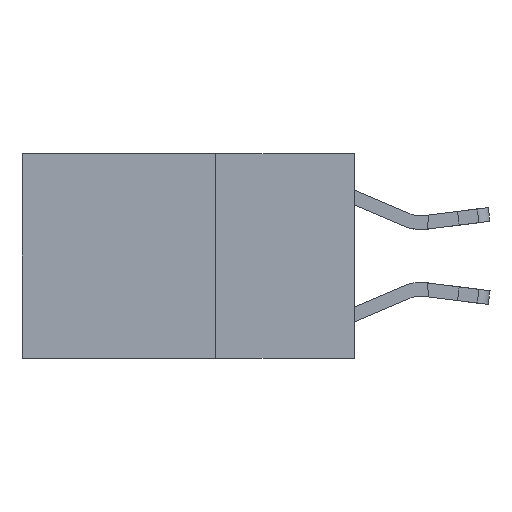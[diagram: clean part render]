
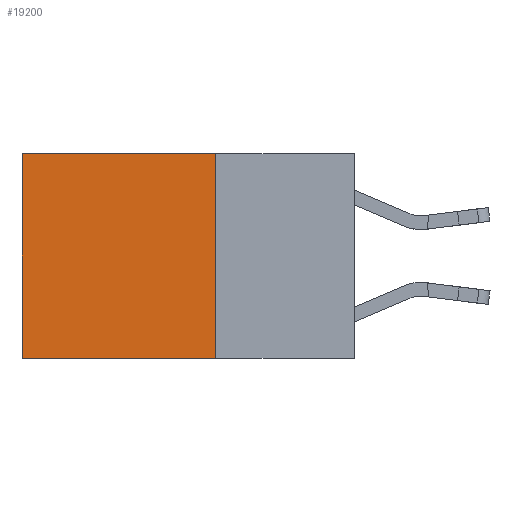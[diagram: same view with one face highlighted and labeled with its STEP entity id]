
A CAD part, left-side view. The second image highlights one B-rep face of the part: STEP entity #19200.
In plain terms, the highlighted planar face has unit normal (-1, 0, 0).
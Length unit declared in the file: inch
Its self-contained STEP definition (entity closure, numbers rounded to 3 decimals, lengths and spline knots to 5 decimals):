
#217 = CARTESIAN_POINT ( 'NONE',  ( 0.2625, 0.6, 0. ) ) ;
#362 = VERTEX_POINT ( 'NONE', #217 ) ;
#408 = VERTEX_POINT ( 'NONE', #25054 ) ;
#1360 = VERTEX_POINT ( 'NONE', #9337 ) ;
#1453 = ORIENTED_EDGE ( 'NONE', *, *, #7594, .F. ) ;
#2041 = CARTESIAN_POINT ( 'NONE',  ( 0.2625, 0.6, 0. ) ) ;
#2956 = DIRECTION ( 'NONE',  ( 0., 1., 0. ) ) ;
#3911 = CARTESIAN_POINT ( 'NONE',  ( 0.2625, 0.25, -0.37 ) ) ;
#4920 = PLANE ( 'NONE',  #14496 ) ;
#5156 = EDGE_CURVE ( 'NONE', #1360, #13276, #16304, .T. ) ;
#5285 = VECTOR ( 'NONE', #17601, 39.37008 ) ;
#6774 = CARTESIAN_POINT ( 'NONE',  ( 0.2625, 0.25, 0. ) ) ;
#6838 = LINE ( 'NONE', #7278, #8966 ) ;
#7278 = CARTESIAN_POINT ( 'NONE',  ( 0.2625, 0.25, 0. ) ) ;
#7594 = EDGE_CURVE ( 'NONE', #408, #1360, #13729, .T. ) ;
#8145 = EDGE_CURVE ( 'NONE', #408, #362, #6838, .T. ) ;
#8325 = ORIENTED_EDGE ( 'NONE', *, *, #8145, .T. ) ;
#8966 = VECTOR ( 'NONE', #2956, 39.37008 ) ;
#8975 = FACE_OUTER_BOUND ( 'NONE', #25027, .T. ) ;
#9202 = DIRECTION ( 'NONE',  ( 0., 1., 0. ) ) ;
#9337 = CARTESIAN_POINT ( 'NONE',  ( 0.2625, 0.25, -0.37 ) ) ;
#11284 = LINE ( 'NONE', #2041, #5285 ) ;
#13276 = VERTEX_POINT ( 'NONE', #14331 ) ;
#13729 = LINE ( 'NONE', #23953, #22444 ) ;
#13831 = DIRECTION ( 'NONE',  ( 0., 0., -1. ) ) ;
#14331 = CARTESIAN_POINT ( 'NONE',  ( 0.2625, 0.6, -0.37 ) ) ;
#14496 = AXIS2_PLACEMENT_3D ( 'NONE', #6774, #27207, #13831 ) ;
#16304 = LINE ( 'NONE', #3911, #20131 ) ;
#17024 = ORIENTED_EDGE ( 'NONE', *, *, #24346, .T. ) ;
#17601 = DIRECTION ( 'NONE',  ( 0., 0., -1. ) ) ;
#19200 = ADVANCED_FACE ( 'NONE', ( #8975 ), #4920, .F. ) ;
#20131 = VECTOR ( 'NONE', #9202, 39.37008 ) ;
#21821 = DIRECTION ( 'NONE',  ( 0., 0., -1. ) ) ;
#22444 = VECTOR ( 'NONE', #21821, 39.37008 ) ;
#23953 = CARTESIAN_POINT ( 'NONE',  ( 0.2625, 0.25, 0. ) ) ;
#24346 = EDGE_CURVE ( 'NONE', #362, #13276, #11284, .T. ) ;
#25027 = EDGE_LOOP ( 'NONE', ( #17024, #27719, #1453, #8325 ) ) ;
#25054 = CARTESIAN_POINT ( 'NONE',  ( 0.2625, 0.25, 0. ) ) ;
#27207 = DIRECTION ( 'NONE',  ( 1., 0., 0. ) ) ;
#27719 = ORIENTED_EDGE ( 'NONE', *, *, #5156, .F. ) ;
